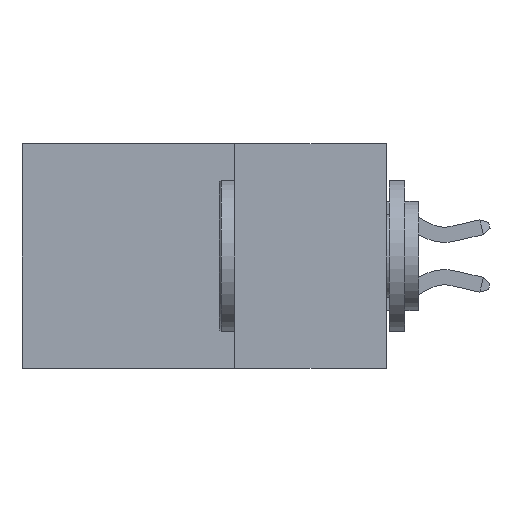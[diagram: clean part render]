
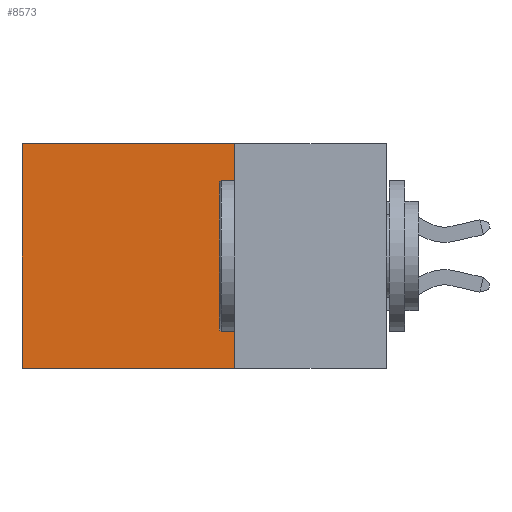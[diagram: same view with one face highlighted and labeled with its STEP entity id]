
A CAD part, left-side view. The second image highlights one B-rep face of the part: STEP entity #8573.
In plain terms, the highlighted planar face has unit normal (-1, 0, 0).
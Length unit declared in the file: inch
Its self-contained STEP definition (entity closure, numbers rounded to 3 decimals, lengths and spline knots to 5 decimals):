
#580 = CARTESIAN_POINT ( 'NONE',  ( 0.2615, 0.25, -0.37 ) ) ;
#844 = ORIENTED_EDGE ( 'NONE', *, *, #18065, .T. ) ;
#1973 = CARTESIAN_POINT ( 'NONE',  ( 0.2615, 0.6, 0. ) ) ;
#1988 = LINE ( 'NONE', #14109, #23632 ) ;
#2942 = CARTESIAN_POINT ( 'NONE',  ( 0.2615, 0.25, -0.37 ) ) ;
#4692 = EDGE_LOOP ( 'NONE', ( #9918, #9226, #15963, #844 ) ) ;
#5134 = DIRECTION ( 'NONE',  ( 0., 0., -1. ) ) ;
#6146 = VERTEX_POINT ( 'NONE', #14998 ) ;
#6344 = AXIS2_PLACEMENT_3D ( 'NONE', #2942, #18089, #5134 ) ;
#7354 = CARTESIAN_POINT ( 'NONE',  ( 0.2615, 0.25, 0. ) ) ;
#7822 = EDGE_CURVE ( 'NONE', #23731, #6146, #9526, .T. ) ;
#8573 = ADVANCED_FACE ( 'NONE', ( #17898 ), #13760, .F. ) ;
#9226 = ORIENTED_EDGE ( 'NONE', *, *, #15224, .F. ) ;
#9302 = LINE ( 'NONE', #7354, #14379 ) ;
#9358 = DIRECTION ( 'NONE',  ( 0., 0., -1. ) ) ;
#9433 = LINE ( 'NONE', #18680, #14501 ) ;
#9526 = LINE ( 'NONE', #580, #13898 ) ;
#9918 = ORIENTED_EDGE ( 'NONE', *, *, #10056, .T. ) ;
#9966 = VERTEX_POINT ( 'NONE', #20456 ) ;
#10056 = EDGE_CURVE ( 'NONE', #11022, #9966, #9433, .T. ) ;
#11022 = VERTEX_POINT ( 'NONE', #1973 ) ;
#13245 = CARTESIAN_POINT ( 'NONE',  ( 0.2615, 0.25, 0. ) ) ;
#13760 = PLANE ( 'NONE',  #6344 ) ;
#13898 = VECTOR ( 'NONE', #9358, 39.37008 ) ;
#14109 = CARTESIAN_POINT ( 'NONE',  ( 0.2615, 0.25, -0.37 ) ) ;
#14379 = VECTOR ( 'NONE', #22497, 39.37008 ) ;
#14501 = VECTOR ( 'NONE', #22898, 39.37008 ) ;
#14998 = CARTESIAN_POINT ( 'NONE',  ( 0.2615, 0.25, -0.37 ) ) ;
#15224 = EDGE_CURVE ( 'NONE', #6146, #9966, #1988, .T. ) ;
#15963 = ORIENTED_EDGE ( 'NONE', *, *, #7822, .F. ) ;
#17898 = FACE_OUTER_BOUND ( 'NONE', #4692, .T. ) ;
#18065 = EDGE_CURVE ( 'NONE', #23731, #11022, #9302, .T. ) ;
#18089 = DIRECTION ( 'NONE',  ( 1., 0., 0. ) ) ;
#18680 = CARTESIAN_POINT ( 'NONE',  ( 0.2615, 0.6, -0.37 ) ) ;
#20456 = CARTESIAN_POINT ( 'NONE',  ( 0.2615, 0.6, -0.37 ) ) ;
#22497 = DIRECTION ( 'NONE',  ( 0., 1., 0. ) ) ;
#22898 = DIRECTION ( 'NONE',  ( 0., 0., -1. ) ) ;
#23632 = VECTOR ( 'NONE', #26929, 39.37008 ) ;
#23731 = VERTEX_POINT ( 'NONE', #13245 ) ;
#26929 = DIRECTION ( 'NONE',  ( 0., 1., 0. ) ) ;
